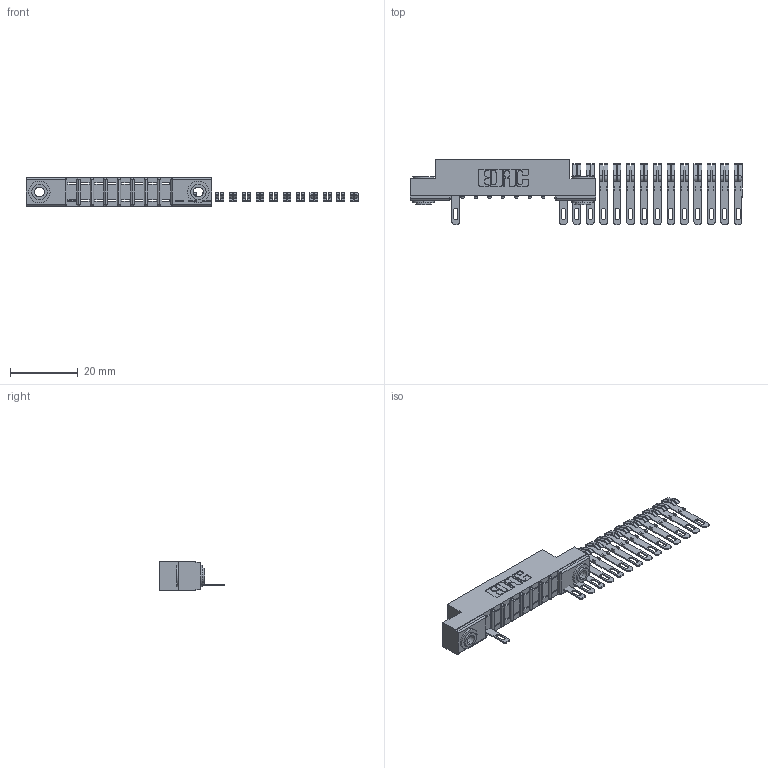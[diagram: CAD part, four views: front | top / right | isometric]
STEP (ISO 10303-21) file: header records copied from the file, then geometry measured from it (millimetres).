
FILE_DESCRIPTION (( 'STEP AP203' ), '1' );
FILE_NAME ('357-022-505-103.STEP', '2018-08-08T21:44:59', ( '' ), ( '' ), 'SwSTEP 2.0', 'SolidWorks 2016', '' );
FILE_SCHEMA (( 'CONFIG_CONTROL_DESIGN' ));
Length unit declared in the file: inch
Products named in the file (4): 357-022-505-103; 307 Part_.156 Dia Mounting Holes; 307-290-001_505; 345-250-002_345-250-002-102
Assembly tree (18 placements, depth 2):
  357-022-505-103
    307 Part_.156 Dia Mounting Holes
    307-290-001_505  x15
    345-250-002_345-250-002-102  x2
Bounding box: 97.83 x 19.18 x 8.71 mm (x, y, z)
Volume: 3612.3 mm3; surface area: 6063.9 mm2
Topology: 18 solids, 18 shells, 879 faces, 2417 edges, 1562 vertices
Faces by surface type: plane 550, cylinder 303, sphere 18, cone 8
Entity records: 12313 total; most frequent: CARTESIAN_POINT 2008, DIRECTION 1997, ORIENTED_EDGE 1978, EDGE_CURVE 989, VECTOR 735, LINE 735, VERTEX_POINT 642, AXIS2_PLACEMENT_3D 631
